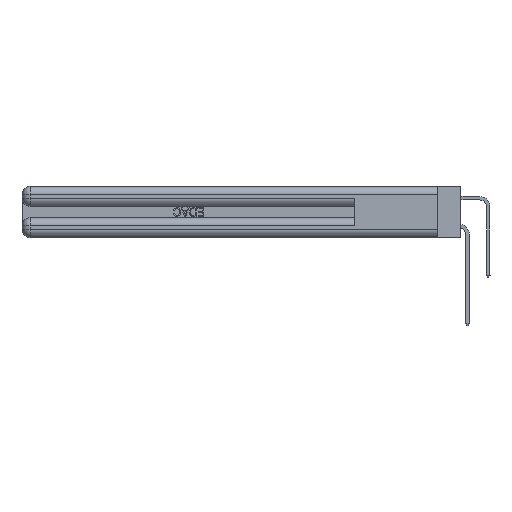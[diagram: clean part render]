
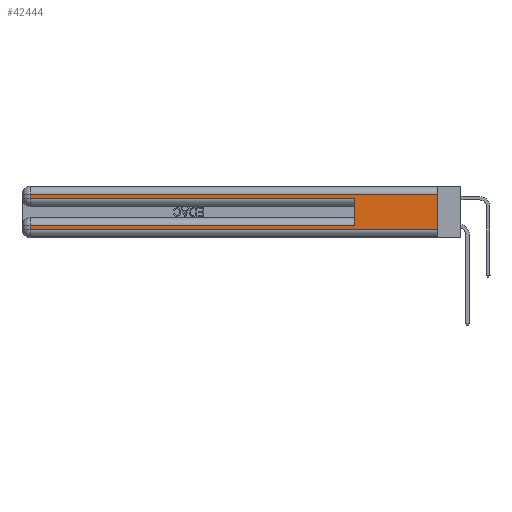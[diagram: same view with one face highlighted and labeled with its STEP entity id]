
A CAD part, left-side view. The second image highlights one B-rep face of the part: STEP entity #42444.
In plain terms, the highlighted planar face has unit normal (-1, 0, 0).
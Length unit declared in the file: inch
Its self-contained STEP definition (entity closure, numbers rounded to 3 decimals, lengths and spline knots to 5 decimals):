
#227 = CARTESIAN_POINT ( 'NONE',  ( 0., 0., 0.285 ) ) ;
#637 = AXIS2_PLACEMENT_3D ( 'NONE', #17311, #5383, #21233 ) ;
#1279 = VECTOR ( 'NONE', #33763, 39.37008 ) ;
#1507 = CARTESIAN_POINT ( 'NONE',  ( 0., 0.6, 0.285 ) ) ;
#2013 = LINE ( 'NONE', #10024, #42699 ) ;
#2419 = CARTESIAN_POINT ( 'NONE',  ( 0., 2.94, 0.085 ) ) ;
#2489 = CARTESIAN_POINT ( 'NONE',  ( 0., 2.94, 0.37 ) ) ;
#2737 = VECTOR ( 'NONE', #12680, 39.37008 ) ;
#4262 = CARTESIAN_POINT ( 'NONE',  ( 0., 2.94, 0.06 ) ) ;
#5383 = DIRECTION ( 'NONE',  ( 1., 0., 0. ) ) ;
#5772 = CARTESIAN_POINT ( 'NONE',  ( 0., 0., 0.06 ) ) ;
#5851 = VERTEX_POINT ( 'NONE', #1507 ) ;
#6123 = EDGE_CURVE ( 'NONE', #22287, #19672, #12292, .T. ) ;
#7247 = DIRECTION ( 'NONE',  ( 0., 0., -1. ) ) ;
#8606 = VERTEX_POINT ( 'NONE', #43831 ) ;
#9407 = CARTESIAN_POINT ( 'NONE',  ( 0., 0., 0.37 ) ) ;
#9433 = EDGE_CURVE ( 'NONE', #35393, #14369, #32664, .T. ) ;
#10024 = CARTESIAN_POINT ( 'NONE',  ( 0., 0.6, 0.145 ) ) ;
#10289 = EDGE_CURVE ( 'NONE', #19672, #14369, #20403, .T. ) ;
#10603 = FACE_OUTER_BOUND ( 'NONE', #32558, .T. ) ;
#12292 = LINE ( 'NONE', #2489, #20242 ) ;
#12455 = ORIENTED_EDGE ( 'NONE', *, *, #18801, .T. ) ;
#12680 = DIRECTION ( 'NONE',  ( 0., -1., 0. ) ) ;
#12830 = CARTESIAN_POINT ( 'NONE',  ( 0., 2.94, 0.285 ) ) ;
#13091 = LINE ( 'NONE', #227, #2737 ) ;
#14369 = VERTEX_POINT ( 'NONE', #5772 ) ;
#14534 = ORIENTED_EDGE ( 'NONE', *, *, #46072, .F. ) ;
#15166 = ORIENTED_EDGE ( 'NONE', *, *, #6123, .T. ) ;
#15498 = VERTEX_POINT ( 'NONE', #26762 ) ;
#16701 = CARTESIAN_POINT ( 'NONE',  ( 0., 0., 0.31 ) ) ;
#16938 = VECTOR ( 'NONE', #32837, 39.37008 ) ;
#17311 = CARTESIAN_POINT ( 'NONE',  ( 0., 0., 0.37 ) ) ;
#18454 = VECTOR ( 'NONE', #45059, 39.37008 ) ;
#18801 = EDGE_CURVE ( 'NONE', #35393, #15498, #40835, .T. ) ;
#19672 = VERTEX_POINT ( 'NONE', #4262 ) ;
#20242 = VECTOR ( 'NONE', #7247, 39.37008 ) ;
#20403 = LINE ( 'NONE', #38979, #29549 ) ;
#20716 = PLANE ( 'NONE',  #637 ) ;
#21079 = VECTOR ( 'NONE', #32568, 39.37008 ) ;
#21233 = DIRECTION ( 'NONE',  ( 0., 0., -1. ) ) ;
#22287 = VERTEX_POINT ( 'NONE', #2419 ) ;
#26762 = CARTESIAN_POINT ( 'NONE',  ( 0., 2.94, 0.31 ) ) ;
#29549 = VECTOR ( 'NONE', #38603, 39.37008 ) ;
#30007 = CARTESIAN_POINT ( 'NONE',  ( 0., 2.94, 0.37 ) ) ;
#32558 = EDGE_LOOP ( 'NONE', ( #49455, #12455, #34638, #48024, #14534, #43152, #15166, #48511 ) ) ;
#32568 = DIRECTION ( 'NONE',  ( 0., 0., -1. ) ) ;
#32664 = LINE ( 'NONE', #9407, #21079 ) ;
#32694 = DIRECTION ( 'NONE',  ( 0., 0., 1. ) ) ;
#32837 = DIRECTION ( 'NONE',  ( 0., 1., 0. ) ) ;
#33763 = DIRECTION ( 'NONE',  ( 0., 1., 0. ) ) ;
#34638 = ORIENTED_EDGE ( 'NONE', *, *, #45520, .T. ) ;
#35393 = VERTEX_POINT ( 'NONE', #41759 ) ;
#35507 = LINE ( 'NONE', #30007, #18454 ) ;
#38603 = DIRECTION ( 'NONE',  ( 0., -1., 0. ) ) ;
#38979 = CARTESIAN_POINT ( 'NONE',  ( 0., 0., 0.06 ) ) ;
#40835 = LINE ( 'NONE', #16701, #1279 ) ;
#41759 = CARTESIAN_POINT ( 'NONE',  ( 0., 0., 0.31 ) ) ;
#42444 = ADVANCED_FACE ( 'NONE', ( #10603 ), #20716, .F. ) ;
#42699 = VECTOR ( 'NONE', #32694, 39.37008 ) ;
#43152 = ORIENTED_EDGE ( 'NONE', *, *, #48891, .T. ) ;
#43831 = CARTESIAN_POINT ( 'NONE',  ( 0., 0.6, 0.085 ) ) ;
#45059 = DIRECTION ( 'NONE',  ( 0., 0., -1. ) ) ;
#45220 = VERTEX_POINT ( 'NONE', #12830 ) ;
#45520 = EDGE_CURVE ( 'NONE', #15498, #45220, #35507, .T. ) ;
#46072 = EDGE_CURVE ( 'NONE', #8606, #5851, #2013, .T. ) ;
#48024 = ORIENTED_EDGE ( 'NONE', *, *, #50301, .T. ) ;
#48511 = ORIENTED_EDGE ( 'NONE', *, *, #10289, .T. ) ;
#48891 = EDGE_CURVE ( 'NONE', #8606, #22287, #49099, .T. ) ;
#49099 = LINE ( 'NONE', #49910, #16938 ) ;
#49455 = ORIENTED_EDGE ( 'NONE', *, *, #9433, .F. ) ;
#49910 = CARTESIAN_POINT ( 'NONE',  ( 0., 0., 0.085 ) ) ;
#50301 = EDGE_CURVE ( 'NONE', #45220, #5851, #13091, .T. ) ;
